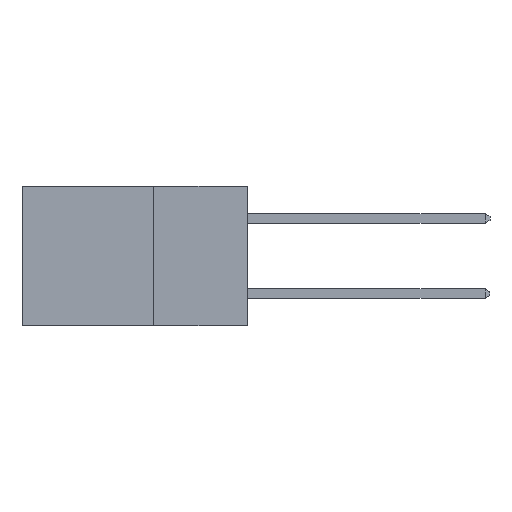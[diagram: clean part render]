
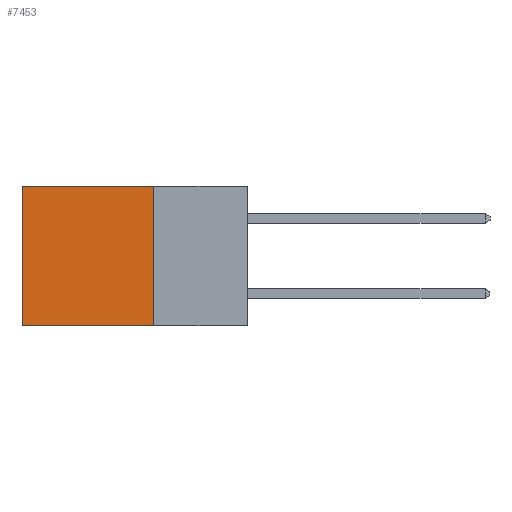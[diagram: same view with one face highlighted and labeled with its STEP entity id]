
A CAD part, left-side view. The second image highlights one B-rep face of the part: STEP entity #7453.
In plain terms, the highlighted planar face has unit normal (-1, 0, 0).
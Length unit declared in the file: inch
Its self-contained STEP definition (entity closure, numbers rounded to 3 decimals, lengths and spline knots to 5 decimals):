
#745 = EDGE_CURVE ( 'NONE', #3577, #15838, #15136, .T. ) ;
#831 = CARTESIAN_POINT ( 'NONE',  ( 0.298, 0.6, 0. ) ) ;
#1009 = CARTESIAN_POINT ( 'NONE',  ( 0.298, 0.6, -0.37 ) ) ;
#1999 = VECTOR ( 'NONE', #7084, 39.37008 ) ;
#2133 = CARTESIAN_POINT ( 'NONE',  ( 0.298, 0.25, -0.37 ) ) ;
#2171 = DIRECTION ( 'NONE',  ( 0., 0., -1. ) ) ;
#3577 = VERTEX_POINT ( 'NONE', #8695 ) ;
#4112 = VECTOR ( 'NONE', #2171, 39.37008 ) ;
#4300 = CARTESIAN_POINT ( 'NONE',  ( 0.298, 0.25, 0. ) ) ;
#4666 = VECTOR ( 'NONE', #9411, 39.37008 ) ;
#4832 = EDGE_LOOP ( 'NONE', ( #9034, #5719, #14448, #14289 ) ) ;
#5036 = LINE ( 'NONE', #15752, #4666 ) ;
#5155 = FACE_OUTER_BOUND ( 'NONE', #4832, .T. ) ;
#5517 = DIRECTION ( 'NONE',  ( 0., 0., -1. ) ) ;
#5717 = LINE ( 'NONE', #2133, #1999 ) ;
#5719 = ORIENTED_EDGE ( 'NONE', *, *, #7632, .F. ) ;
#7084 = DIRECTION ( 'NONE',  ( 0., 1., 0. ) ) ;
#7453 = ADVANCED_FACE ( 'NONE', ( #5155 ), #10701, .F. ) ;
#7632 = EDGE_CURVE ( 'NONE', #14357, #7745, #5717, .T. ) ;
#7745 = VERTEX_POINT ( 'NONE', #1009 ) ;
#7868 = VECTOR ( 'NONE', #15010, 39.37008 ) ;
#7886 = AXIS2_PLACEMENT_3D ( 'NONE', #4300, #13190, #5517 ) ;
#8695 = CARTESIAN_POINT ( 'NONE',  ( 0.298, 0.25, 0. ) ) ;
#9034 = ORIENTED_EDGE ( 'NONE', *, *, #15636, .T. ) ;
#9411 = DIRECTION ( 'NONE',  ( 0., 0., -1. ) ) ;
#10701 = PLANE ( 'NONE',  #7886 ) ;
#11216 = EDGE_CURVE ( 'NONE', #3577, #14357, #5036, .T. ) ;
#12664 = CARTESIAN_POINT ( 'NONE',  ( 0.298, 0.6, 0. ) ) ;
#12830 = CARTESIAN_POINT ( 'NONE',  ( 0.298, 0.25, -0.37 ) ) ;
#13190 = DIRECTION ( 'NONE',  ( 1., 0., 0. ) ) ;
#14254 = LINE ( 'NONE', #831, #4112 ) ;
#14289 = ORIENTED_EDGE ( 'NONE', *, *, #745, .T. ) ;
#14357 = VERTEX_POINT ( 'NONE', #12830 ) ;
#14448 = ORIENTED_EDGE ( 'NONE', *, *, #11216, .F. ) ;
#15010 = DIRECTION ( 'NONE',  ( 0., 1., 0. ) ) ;
#15032 = CARTESIAN_POINT ( 'NONE',  ( 0.298, 0.25, 0. ) ) ;
#15136 = LINE ( 'NONE', #15032, #7868 ) ;
#15636 = EDGE_CURVE ( 'NONE', #15838, #7745, #14254, .T. ) ;
#15752 = CARTESIAN_POINT ( 'NONE',  ( 0.298, 0.25, 0. ) ) ;
#15838 = VERTEX_POINT ( 'NONE', #12664 ) ;
